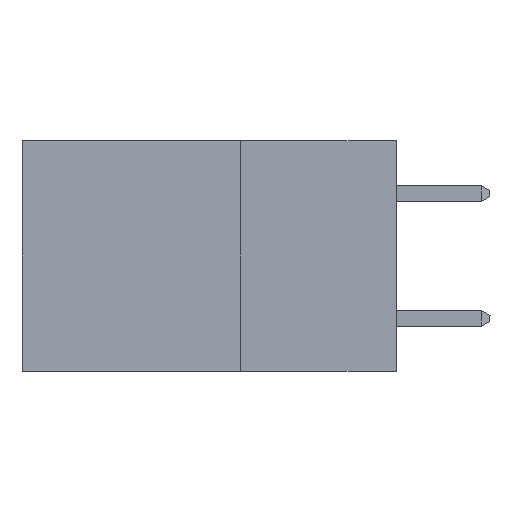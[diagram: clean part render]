
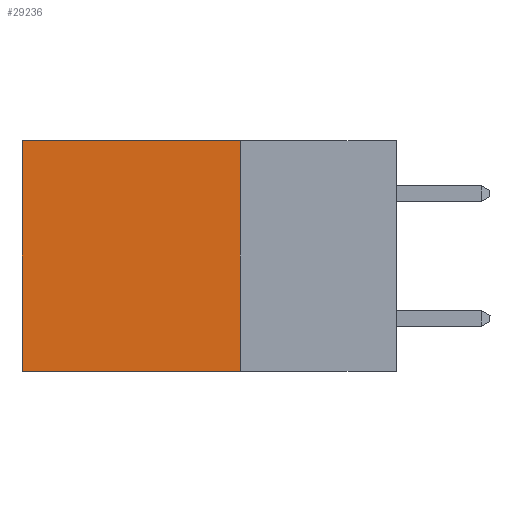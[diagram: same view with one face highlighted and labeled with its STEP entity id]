
A CAD part, left-side view. The second image highlights one B-rep face of the part: STEP entity #29236.
In plain terms, the highlighted planar face has unit normal (-1, 0, 0).
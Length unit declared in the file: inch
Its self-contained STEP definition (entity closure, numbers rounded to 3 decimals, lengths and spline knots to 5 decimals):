
#886 = CARTESIAN_POINT ( 'NONE',  ( 0.298, 0.25, 0. ) ) ;
#1436 = DIRECTION ( 'NONE',  ( 0., 0., -1. ) ) ;
#1652 = CARTESIAN_POINT ( 'NONE',  ( 0.298, 0.25, -0.37 ) ) ;
#1660 = FACE_OUTER_BOUND ( 'NONE', #24078, .T. ) ;
#2272 = DIRECTION ( 'NONE',  ( 1., 0., 0. ) ) ;
#2860 = VERTEX_POINT ( 'NONE', #23288 ) ;
#3170 = VERTEX_POINT ( 'NONE', #10829 ) ;
#3872 = VECTOR ( 'NONE', #5781, 39.37008 ) ;
#5538 = CARTESIAN_POINT ( 'NONE',  ( 0.298, 0.25, 0. ) ) ;
#5781 = DIRECTION ( 'NONE',  ( 0., 0., -1. ) ) ;
#8828 = LINE ( 'NONE', #15391, #27172 ) ;
#10829 = CARTESIAN_POINT ( 'NONE',  ( 0.298, 0.6, -0.37 ) ) ;
#11273 = DIRECTION ( 'NONE',  ( 0., 1., 0. ) ) ;
#11616 = VERTEX_POINT ( 'NONE', #25069 ) ;
#12140 = AXIS2_PLACEMENT_3D ( 'NONE', #16268, #2272, #18590 ) ;
#14603 = ORIENTED_EDGE ( 'NONE', *, *, #29573, .F. ) ;
#14879 = EDGE_CURVE ( 'NONE', #2860, #3170, #8828, .T. ) ;
#15391 = CARTESIAN_POINT ( 'NONE',  ( 0.298, 0.6, 0. ) ) ;
#15968 = EDGE_CURVE ( 'NONE', #11616, #2860, #20713, .T. ) ;
#16268 = CARTESIAN_POINT ( 'NONE',  ( 0.298, 0.25, 0. ) ) ;
#17885 = ORIENTED_EDGE ( 'NONE', *, *, #24203, .F. ) ;
#18050 = LINE ( 'NONE', #22747, #21975 ) ;
#18590 = DIRECTION ( 'NONE',  ( 0., 0., -1. ) ) ;
#19989 = VECTOR ( 'NONE', #24054, 39.37008 ) ;
#20713 = LINE ( 'NONE', #5538, #19989 ) ;
#20939 = ORIENTED_EDGE ( 'NONE', *, *, #15968, .T. ) ;
#21975 = VECTOR ( 'NONE', #11273, 39.37008 ) ;
#22747 = CARTESIAN_POINT ( 'NONE',  ( 0.298, 0.25, -0.37 ) ) ;
#22817 = VERTEX_POINT ( 'NONE', #1652 ) ;
#23099 = PLANE ( 'NONE',  #12140 ) ;
#23288 = CARTESIAN_POINT ( 'NONE',  ( 0.298, 0.6, 0. ) ) ;
#24054 = DIRECTION ( 'NONE',  ( 0., 1., 0. ) ) ;
#24078 = EDGE_LOOP ( 'NONE', ( #29709, #17885, #14603, #20939 ) ) ;
#24203 = EDGE_CURVE ( 'NONE', #22817, #3170, #18050, .T. ) ;
#25069 = CARTESIAN_POINT ( 'NONE',  ( 0.298, 0.25, 0. ) ) ;
#27172 = VECTOR ( 'NONE', #1436, 39.37008 ) ;
#29188 = LINE ( 'NONE', #886, #3872 ) ;
#29236 = ADVANCED_FACE ( 'NONE', ( #1660 ), #23099, .F. ) ;
#29573 = EDGE_CURVE ( 'NONE', #11616, #22817, #29188, .T. ) ;
#29709 = ORIENTED_EDGE ( 'NONE', *, *, #14879, .T. ) ;
